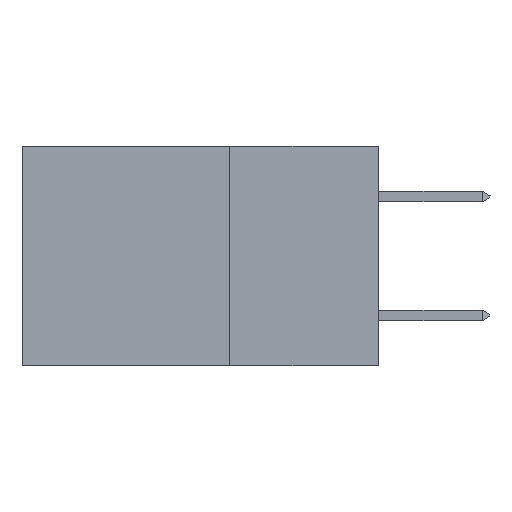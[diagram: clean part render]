
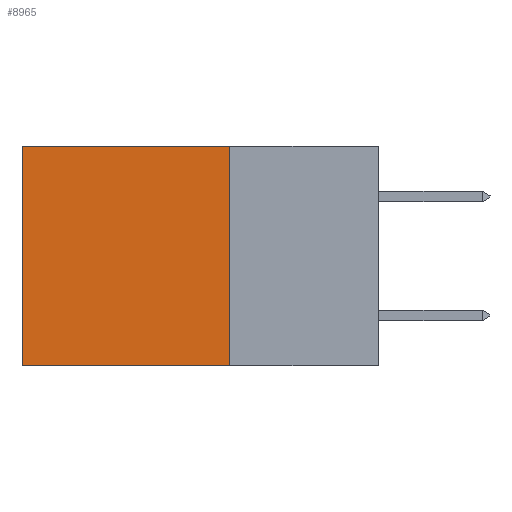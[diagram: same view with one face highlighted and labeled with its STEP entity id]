
A CAD part, left-side view. The second image highlights one B-rep face of the part: STEP entity #8965.
In plain terms, the highlighted planar face has unit normal (-1, 0, 0).
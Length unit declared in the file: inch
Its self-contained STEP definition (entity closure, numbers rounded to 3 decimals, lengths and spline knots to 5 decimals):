
#880 = EDGE_CURVE ( 'NONE', #9808, #15327, #14403, .T. ) ;
#1106 = CARTESIAN_POINT ( 'NONE',  ( 0.2615, 0.6, -0.37 ) ) ;
#1562 = VECTOR ( 'NONE', #5680, 39.37008 ) ;
#2623 = CARTESIAN_POINT ( 'NONE',  ( 0.2615, 0.6, 0. ) ) ;
#2886 = DIRECTION ( 'NONE',  ( 0., 0., -1. ) ) ;
#3794 = EDGE_LOOP ( 'NONE', ( #18339, #18597, #6419, #9061 ) ) ;
#4184 = LINE ( 'NONE', #10689, #1562 ) ;
#4217 = DIRECTION ( 'NONE',  ( 1., 0., 0. ) ) ;
#4434 = CARTESIAN_POINT ( 'NONE',  ( 0.2615, 0.25, -0.37 ) ) ;
#5230 = VERTEX_POINT ( 'NONE', #7838 ) ;
#5680 = DIRECTION ( 'NONE',  ( 0., 0., -1. ) ) ;
#6046 = PLANE ( 'NONE',  #10645 ) ;
#6419 = ORIENTED_EDGE ( 'NONE', *, *, #19707, .F. ) ;
#6959 = CARTESIAN_POINT ( 'NONE',  ( 0.2615, 0.25, -0.37 ) ) ;
#7700 = DIRECTION ( 'NONE',  ( 0., 1., 0. ) ) ;
#7838 = CARTESIAN_POINT ( 'NONE',  ( 0.2615, 0.25, 0. ) ) ;
#8503 = VECTOR ( 'NONE', #7700, 39.37008 ) ;
#8718 = LINE ( 'NONE', #20168, #21266 ) ;
#8965 = ADVANCED_FACE ( 'NONE', ( #17495 ), #6046, .F. ) ;
#9061 = ORIENTED_EDGE ( 'NONE', *, *, #20618, .T. ) ;
#9314 = LINE ( 'NONE', #15975, #8503 ) ;
#9808 = VERTEX_POINT ( 'NONE', #2623 ) ;
#10645 = AXIS2_PLACEMENT_3D ( 'NONE', #4434, #4217, #11054 ) ;
#10689 = CARTESIAN_POINT ( 'NONE',  ( 0.2615, 0.25, -0.37 ) ) ;
#10904 = CARTESIAN_POINT ( 'NONE',  ( 0.2615, 0.6, -0.37 ) ) ;
#11054 = DIRECTION ( 'NONE',  ( 0., 0., -1. ) ) ;
#11313 = VERTEX_POINT ( 'NONE', #6959 ) ;
#14403 = LINE ( 'NONE', #10904, #14572 ) ;
#14572 = VECTOR ( 'NONE', #2886, 39.37008 ) ;
#15327 = VERTEX_POINT ( 'NONE', #1106 ) ;
#15975 = CARTESIAN_POINT ( 'NONE',  ( 0.2615, 0.25, 0. ) ) ;
#16571 = EDGE_CURVE ( 'NONE', #11313, #15327, #8718, .T. ) ;
#16796 = DIRECTION ( 'NONE',  ( 0., 1., 0. ) ) ;
#17495 = FACE_OUTER_BOUND ( 'NONE', #3794, .T. ) ;
#18339 = ORIENTED_EDGE ( 'NONE', *, *, #880, .T. ) ;
#18597 = ORIENTED_EDGE ( 'NONE', *, *, #16571, .F. ) ;
#19707 = EDGE_CURVE ( 'NONE', #5230, #11313, #4184, .T. ) ;
#20168 = CARTESIAN_POINT ( 'NONE',  ( 0.2615, 0.25, -0.37 ) ) ;
#20618 = EDGE_CURVE ( 'NONE', #5230, #9808, #9314, .T. ) ;
#21266 = VECTOR ( 'NONE', #16796, 39.37008 ) ;
